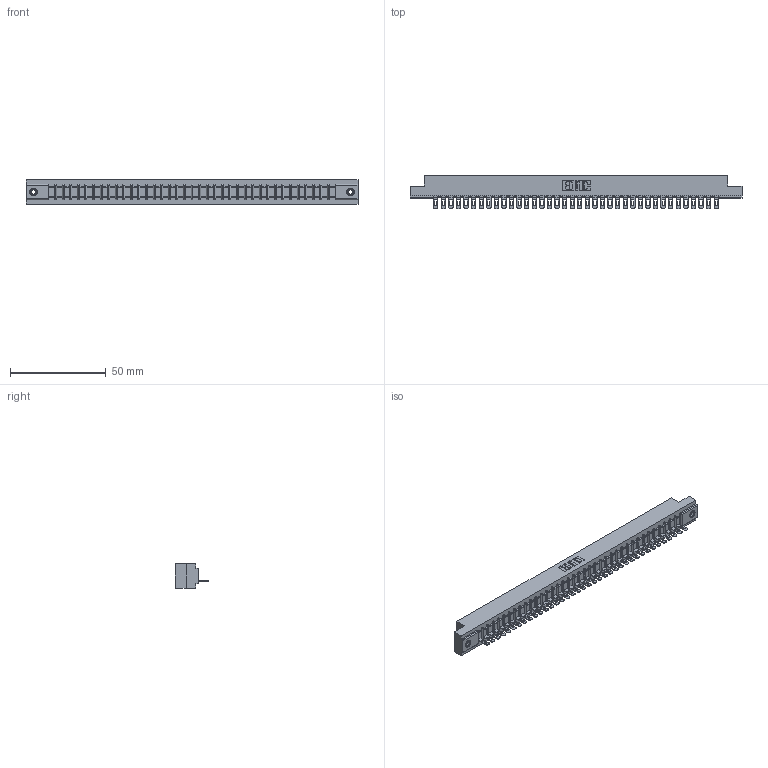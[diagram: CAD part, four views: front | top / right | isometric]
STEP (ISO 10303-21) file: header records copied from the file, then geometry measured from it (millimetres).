
FILE_DESCRIPTION (( 'STEP AP203' ), '1' );
FILE_NAME ('307-038-501-108.STEP', '2019-09-05T08:53:28', ( '' ), ( '' ), 'SwSTEP 2.0', 'SolidWorks 2016', '' );
FILE_SCHEMA (( 'CONFIG_CONTROL_DESIGN' ));
Length unit declared in the file: inch
Products named in the file (4): 307-290-002_501; 307-038-501-108; 307 Part_.156 Dia Mounting Holes; 345-250-001_345-250-003-102
Assembly tree (41 placements, depth 2):
  307-038-501-108
    307 Part_.156 Dia Mounting Holes
    307-290-002_501  x38
    345-250-001_345-250-003-102  x2
Bounding box: 173.58 x 17.42 x 12.7 mm (x, y, z)
Volume: 18572.4 mm3; surface area: 23540.8 mm2
Topology: 41 solids, 41 shells, 3105 faces, 9503 edges, 6222 vertices
Faces by surface type: plane 1774, cylinder 1237, sphere 78, cone 12, torus 4
Entity records: 35049 total; most frequent: CARTESIAN_POINT 5891, ORIENTED_EDGE 5874, DIRECTION 5739, EDGE_CURVE 2937, LINE 2243, VECTOR 2243, VERTEX_POINT 1900, AXIS2_PLACEMENT_3D 1748
